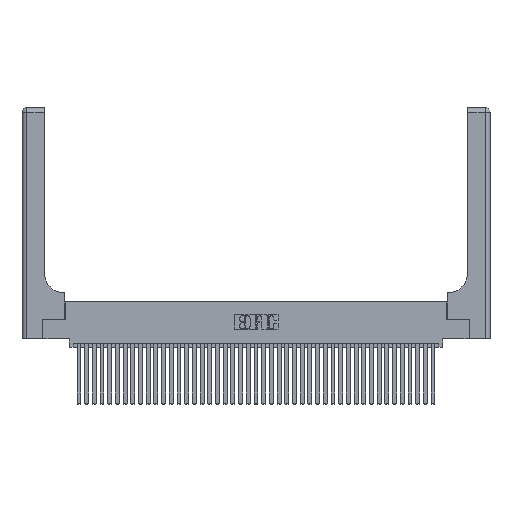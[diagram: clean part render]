
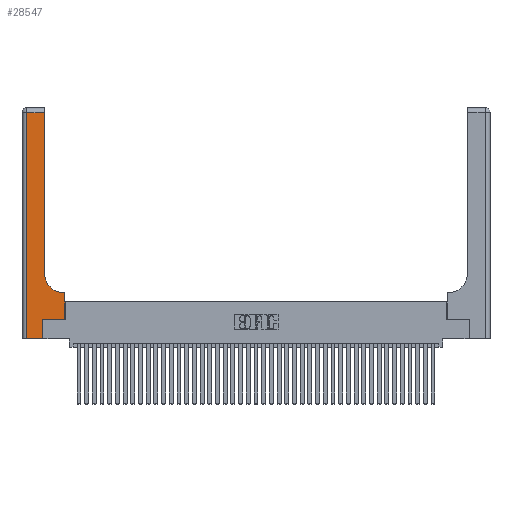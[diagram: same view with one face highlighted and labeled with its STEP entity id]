
A CAD part, top view. The second image highlights one B-rep face of the part: STEP entity #28547.
In plain terms, the highlighted planar face has unit normal (0, 0, 1).
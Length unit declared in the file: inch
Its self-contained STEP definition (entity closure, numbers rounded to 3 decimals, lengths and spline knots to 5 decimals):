
#141 = ORIENTED_EDGE ( 'NONE', *, *, #2142, .T. ) ;
#1470 = VERTEX_POINT ( 'NONE', #16675 ) ;
#1482 = LINE ( 'NONE', #36571, #24458 ) ;
#1851 = LINE ( 'NONE', #19378, #27330 ) ;
#2035 = EDGE_CURVE ( 'NONE', #1470, #2682, #11521, .T. ) ;
#2142 = EDGE_CURVE ( 'NONE', #37150, #27642, #24517, .T. ) ;
#2256 = LINE ( 'NONE', #19553, #35224 ) ;
#2682 = VERTEX_POINT ( 'NONE', #18168 ) ;
#2955 = EDGE_CURVE ( 'NONE', #25288, #37150, #32027, .T. ) ;
#4390 = CARTESIAN_POINT ( 'NONE',  ( 0., 3., 0.37 ) ) ;
#4799 = CARTESIAN_POINT ( 'NONE',  ( 0., 0., 0.37 ) ) ;
#7532 = EDGE_CURVE ( 'NONE', #2682, #14257, #1482, .T. ) ;
#8452 = DIRECTION ( 'NONE',  ( 0., 0., -1. ) ) ;
#8870 = CARTESIAN_POINT ( 'NONE',  ( 0.5415, 0.85, 0.37 ) ) ;
#9043 = EDGE_CURVE ( 'NONE', #27642, #28215, #1851, .T. ) ;
#9228 = CARTESIAN_POINT ( 'NONE',  ( 0.2915, 3., 0.37 ) ) ;
#9288 = CARTESIAN_POINT ( 'NONE',  ( 0.06, 2.94, 0.37 ) ) ;
#9739 = VECTOR ( 'NONE', #36957, 39.37008 ) ;
#10489 = DIRECTION ( 'NONE',  ( 1., 0., 0. ) ) ;
#11521 = LINE ( 'NONE', #38457, #26509 ) ;
#13368 = ORIENTED_EDGE ( 'NONE', *, *, #32346, .T. ) ;
#14257 = VERTEX_POINT ( 'NONE', #16768 ) ;
#14454 = CARTESIAN_POINT ( 'NONE',  ( 0.06, 3., 0.37 ) ) ;
#14694 = DIRECTION ( 'NONE',  ( 0., 1., 0. ) ) ;
#14890 = LINE ( 'NONE', #19184, #30362 ) ;
#14895 = DIRECTION ( 'NONE',  ( 1., 0., 0. ) ) ;
#15776 = CARTESIAN_POINT ( 'NONE',  ( 0.2915, 2.94, 0.37 ) ) ;
#16611 = DIRECTION ( 'NONE',  ( 0., 1., 0. ) ) ;
#16675 = CARTESIAN_POINT ( 'NONE',  ( 0.269, 0.25, 0.37 ) ) ;
#16768 = CARTESIAN_POINT ( 'NONE',  ( 0.5585, 0.6, 0.37 ) ) ;
#16777 = EDGE_LOOP ( 'NONE', ( #141, #25896, #32100, #13368, #19904, #22298, #21988, #24807, #22514 ) ) ;
#16923 = VERTEX_POINT ( 'NONE', #40863 ) ;
#18168 = CARTESIAN_POINT ( 'NONE',  ( 0.5585, 0.25, 0.37 ) ) ;
#18580 = EDGE_CURVE ( 'NONE', #28215, #24070, #29085, .T. ) ;
#19184 = CARTESIAN_POINT ( 'NONE',  ( 0.2915, 0.6, 0.37 ) ) ;
#19344 = AXIS2_PLACEMENT_3D ( 'NONE', #8870, #8452, #14895 ) ;
#19378 = CARTESIAN_POINT ( 'NONE',  ( 0., 2.94, 0.37 ) ) ;
#19459 = DIRECTION ( 'NONE',  ( -1., 0., 0. ) ) ;
#19553 = CARTESIAN_POINT ( 'NONE',  ( 0.269, 0., 0.37 ) ) ;
#19904 = ORIENTED_EDGE ( 'NONE', *, *, #32723, .T. ) ;
#20870 = CARTESIAN_POINT ( 'NONE',  ( 0.5415, 0.6, 0.37 ) ) ;
#21988 = ORIENTED_EDGE ( 'NONE', *, *, #7532, .T. ) ;
#22298 = ORIENTED_EDGE ( 'NONE', *, *, #2035, .T. ) ;
#22514 = ORIENTED_EDGE ( 'NONE', *, *, #2955, .T. ) ;
#22924 = AXIS2_PLACEMENT_3D ( 'NONE', #4390, #30232, #33289 ) ;
#23249 = CARTESIAN_POINT ( 'NONE',  ( 0.2915, 0.85, 0.37 ) ) ;
#23478 = CARTESIAN_POINT ( 'NONE',  ( 0.06, 0., 0.37 ) ) ;
#24070 = VERTEX_POINT ( 'NONE', #23478 ) ;
#24458 = VECTOR ( 'NONE', #27197, 39.37008 ) ;
#24517 = LINE ( 'NONE', #9228, #36030 ) ;
#24807 = ORIENTED_EDGE ( 'NONE', *, *, #30358, .T. ) ;
#25288 = VERTEX_POINT ( 'NONE', #20870 ) ;
#25896 = ORIENTED_EDGE ( 'NONE', *, *, #9043, .T. ) ;
#26509 = VECTOR ( 'NONE', #10489, 39.37008 ) ;
#27197 = DIRECTION ( 'NONE',  ( 0., 1., 0. ) ) ;
#27214 = FACE_OUTER_BOUND ( 'NONE', #16777, .T. ) ;
#27330 = VECTOR ( 'NONE', #36145, 39.37008 ) ;
#27642 = VERTEX_POINT ( 'NONE', #15776 ) ;
#28215 = VERTEX_POINT ( 'NONE', #9288 ) ;
#28547 = ADVANCED_FACE ( 'NONE', ( #27214 ), #39423, .F. ) ;
#29085 = LINE ( 'NONE', #14454, #36082 ) ;
#30232 = DIRECTION ( 'NONE',  ( 0., 0., -1. ) ) ;
#30358 = EDGE_CURVE ( 'NONE', #14257, #25288, #14890, .T. ) ;
#30362 = VECTOR ( 'NONE', #19459, 39.37008 ) ;
#32027 = CIRCLE ( 'NONE', #19344, 0.25 ) ;
#32100 = ORIENTED_EDGE ( 'NONE', *, *, #18580, .T. ) ;
#32346 = EDGE_CURVE ( 'NONE', #24070, #16923, #32761, .T. ) ;
#32723 = EDGE_CURVE ( 'NONE', #16923, #1470, #2256, .T. ) ;
#32761 = LINE ( 'NONE', #4799, #9739 ) ;
#33289 = DIRECTION ( 'NONE',  ( -1., 0., 0. ) ) ;
#35224 = VECTOR ( 'NONE', #14694, 39.37008 ) ;
#36030 = VECTOR ( 'NONE', #16611, 39.37008 ) ;
#36082 = VECTOR ( 'NONE', #40131, 39.37008 ) ;
#36145 = DIRECTION ( 'NONE',  ( -1., 0., 0. ) ) ;
#36571 = CARTESIAN_POINT ( 'NONE',  ( 0.5585, 0.25, 0.37 ) ) ;
#36957 = DIRECTION ( 'NONE',  ( 1., 0., 0. ) ) ;
#37150 = VERTEX_POINT ( 'NONE', #23249 ) ;
#38457 = CARTESIAN_POINT ( 'NONE',  ( 0.269, 0.25, 0.37 ) ) ;
#39423 = PLANE ( 'NONE',  #22924 ) ;
#40131 = DIRECTION ( 'NONE',  ( 0., -1., 0. ) ) ;
#40863 = CARTESIAN_POINT ( 'NONE',  ( 0.269, 0., 0.37 ) ) ;
